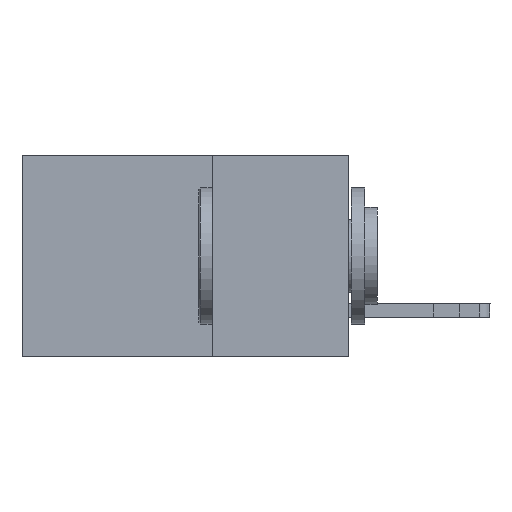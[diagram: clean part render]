
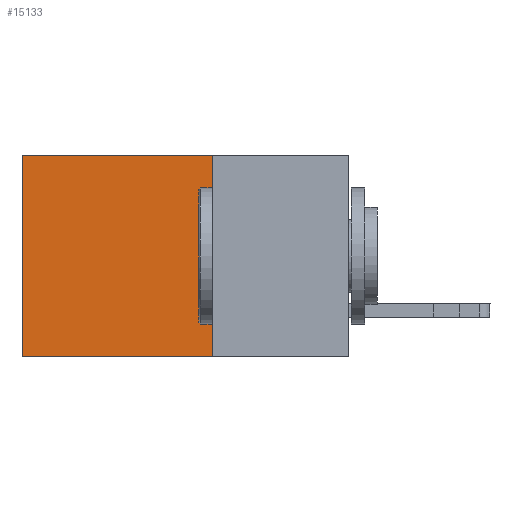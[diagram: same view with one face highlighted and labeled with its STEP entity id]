
A CAD part, left-side view. The second image highlights one B-rep face of the part: STEP entity #15133.
In plain terms, the highlighted planar face has unit normal (-1, 0, 0).
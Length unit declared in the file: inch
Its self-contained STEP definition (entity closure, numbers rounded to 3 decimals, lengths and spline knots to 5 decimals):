
#62 = CARTESIAN_POINT ( 'NONE',  ( 0.2615, 0.25, -0.37 ) ) ;
#576 = LINE ( 'NONE', #4678, #13960 ) ;
#624 = DIRECTION ( 'NONE',  ( 0., 0., -1. ) ) ;
#1262 = EDGE_CURVE ( 'NONE', #7740, #16303, #16573, .T. ) ;
#1372 = DIRECTION ( 'NONE',  ( 0., 0., -1. ) ) ;
#1967 = EDGE_CURVE ( 'NONE', #16303, #9312, #8132, .T. ) ;
#2070 = EDGE_CURVE ( 'NONE', #7740, #14065, #9502, .T. ) ;
#3000 = VECTOR ( 'NONE', #624, 39.37008 ) ;
#3227 = CARTESIAN_POINT ( 'NONE',  ( 0.2615, 0.6, -0.37 ) ) ;
#3504 = CARTESIAN_POINT ( 'NONE',  ( 0.2615, 0.25, -0.37 ) ) ;
#4625 = ORIENTED_EDGE ( 'NONE', *, *, #1967, .F. ) ;
#4678 = CARTESIAN_POINT ( 'NONE',  ( 0.2615, 0.6, -0.37 ) ) ;
#7740 = VERTEX_POINT ( 'NONE', #8290 ) ;
#7968 = PLANE ( 'NONE',  #8418 ) ;
#8132 = LINE ( 'NONE', #13978, #10691 ) ;
#8290 = CARTESIAN_POINT ( 'NONE',  ( 0.2615, 0.25, 0. ) ) ;
#8418 = AXIS2_PLACEMENT_3D ( 'NONE', #62, #9249, #1372 ) ;
#8603 = EDGE_LOOP ( 'NONE', ( #14491, #4625, #9105, #16331 ) ) ;
#9105 = ORIENTED_EDGE ( 'NONE', *, *, #1262, .F. ) ;
#9249 = DIRECTION ( 'NONE',  ( 1., 0., 0. ) ) ;
#9312 = VERTEX_POINT ( 'NONE', #3227 ) ;
#9502 = LINE ( 'NONE', #16023, #12109 ) ;
#10018 = DIRECTION ( 'NONE',  ( 0., 1., 0. ) ) ;
#10691 = VECTOR ( 'NONE', #11177, 39.37008 ) ;
#10784 = FACE_OUTER_BOUND ( 'NONE', #8603, .T. ) ;
#10872 = CARTESIAN_POINT ( 'NONE',  ( 0.2615, 0.6, 0. ) ) ;
#11177 = DIRECTION ( 'NONE',  ( 0., 1., 0. ) ) ;
#12109 = VECTOR ( 'NONE', #10018, 39.37008 ) ;
#13805 = CARTESIAN_POINT ( 'NONE',  ( 0.2615, 0.25, -0.37 ) ) ;
#13960 = VECTOR ( 'NONE', #14894, 39.37008 ) ;
#13978 = CARTESIAN_POINT ( 'NONE',  ( 0.2615, 0.25, -0.37 ) ) ;
#14065 = VERTEX_POINT ( 'NONE', #10872 ) ;
#14197 = EDGE_CURVE ( 'NONE', #14065, #9312, #576, .T. ) ;
#14491 = ORIENTED_EDGE ( 'NONE', *, *, #14197, .T. ) ;
#14894 = DIRECTION ( 'NONE',  ( 0., 0., -1. ) ) ;
#15133 = ADVANCED_FACE ( 'NONE', ( #10784 ), #7968, .F. ) ;
#16023 = CARTESIAN_POINT ( 'NONE',  ( 0.2615, 0.25, 0. ) ) ;
#16303 = VERTEX_POINT ( 'NONE', #3504 ) ;
#16331 = ORIENTED_EDGE ( 'NONE', *, *, #2070, .T. ) ;
#16573 = LINE ( 'NONE', #13805, #3000 ) ;
